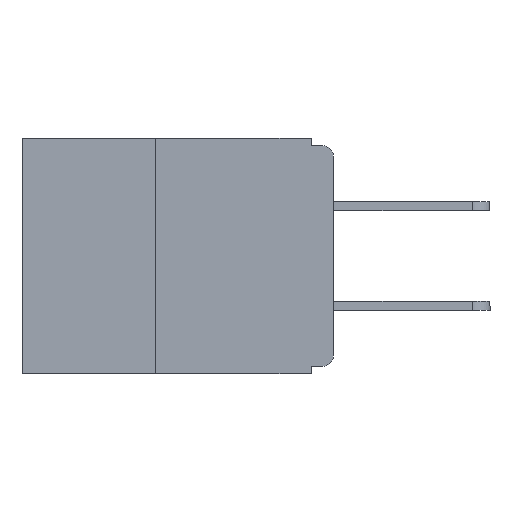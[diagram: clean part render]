
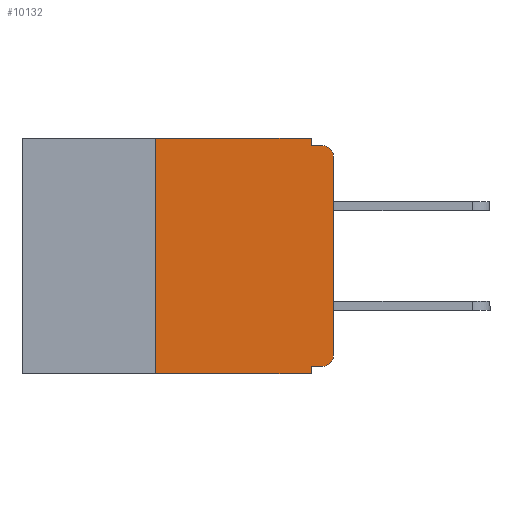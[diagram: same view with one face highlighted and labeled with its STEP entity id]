
A CAD part, left-side view. The second image highlights one B-rep face of the part: STEP entity #10132.
In plain terms, the highlighted planar face has unit normal (-1, 0, 0).
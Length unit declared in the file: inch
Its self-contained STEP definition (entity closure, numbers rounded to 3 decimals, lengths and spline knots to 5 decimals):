
#127 = LINE ( 'NONE', #15783, #6405 ) ;
#348 = VERTEX_POINT ( 'NONE', #14141 ) ;
#1384 = LINE ( 'NONE', #26669, #18188 ) ;
#2571 = CIRCLE ( 'NONE', #19677, 0.015 ) ;
#2648 = VERTEX_POINT ( 'NONE', #5834 ) ;
#2843 = DIRECTION ( 'NONE',  ( 1., 0., 0. ) ) ;
#3159 = EDGE_CURVE ( 'NONE', #17202, #8400, #13099, .T. ) ;
#3169 = AXIS2_PLACEMENT_3D ( 'NONE', #24977, #12440, #27015 ) ;
#4123 = DIRECTION ( 'NONE',  ( 0., 0., 1. ) ) ;
#4272 = LINE ( 'NONE', #15390, #20391 ) ;
#5052 = LINE ( 'NONE', #18734, #15496 ) ;
#5368 = DIRECTION ( 'NONE',  ( 0., -1., 0. ) ) ;
#5501 = CARTESIAN_POINT ( 'NONE',  ( 0., 0.031, -0.32 ) ) ;
#5834 = CARTESIAN_POINT ( 'NONE',  ( 0., 0.015, -0.32 ) ) ;
#6405 = VECTOR ( 'NONE', #5368, 39.37008 ) ;
#6448 = EDGE_CURVE ( 'NONE', #2648, #16755, #1384, .T. ) ;
#6973 = DIRECTION ( 'NONE',  ( 0., 0., -1. ) ) ;
#7498 = ORIENTED_EDGE ( 'NONE', *, *, #3159, .T. ) ;
#7514 = VERTEX_POINT ( 'NONE', #11996 ) ;
#7609 = ORIENTED_EDGE ( 'NONE', *, *, #23873, .T. ) ;
#7695 = CARTESIAN_POINT ( 'NONE',  ( 0., 0.031, 0. ) ) ;
#8369 = ORIENTED_EDGE ( 'NONE', *, *, #14883, .F. ) ;
#8400 = VERTEX_POINT ( 'NONE', #19944 ) ;
#8676 = DIRECTION ( 'NONE',  ( -1., 0., 0. ) ) ;
#9037 = CARTESIAN_POINT ( 'NONE',  ( 0., 0.437, 0. ) ) ;
#9240 = ORIENTED_EDGE ( 'NONE', *, *, #21764, .F. ) ;
#9447 = VECTOR ( 'NONE', #22319, 39.37008 ) ;
#9694 = ORIENTED_EDGE ( 'NONE', *, *, #19086, .F. ) ;
#10132 = ADVANCED_FACE ( 'NONE', ( #12997 ), #15371, .F. ) ;
#10397 = ORIENTED_EDGE ( 'NONE', *, *, #17545, .F. ) ;
#10726 = ORIENTED_EDGE ( 'NONE', *, *, #16083, .T. ) ;
#10773 = VERTEX_POINT ( 'NONE', #19555 ) ;
#11553 = CARTESIAN_POINT ( 'NONE',  ( 0., 0.437, 0. ) ) ;
#11996 = CARTESIAN_POINT ( 'NONE',  ( 0., 0.25, 0. ) ) ;
#12440 = DIRECTION ( 'NONE',  ( -1., 0., 0. ) ) ;
#12457 = ORIENTED_EDGE ( 'NONE', *, *, #14672, .F. ) ;
#12593 = ORIENTED_EDGE ( 'NONE', *, *, #6448, .F. ) ;
#12857 = ORIENTED_EDGE ( 'NONE', *, *, #21117, .T. ) ;
#12874 = CARTESIAN_POINT ( 'NONE',  ( 0., 0.031, 0. ) ) ;
#12969 = DIRECTION ( 'NONE',  ( 0., 0., -1. ) ) ;
#12997 = FACE_OUTER_BOUND ( 'NONE', #22557, .T. ) ;
#13099 = LINE ( 'NONE', #14351, #23636 ) ;
#13327 = VECTOR ( 'NONE', #12969, 39.37008 ) ;
#13436 = CARTESIAN_POINT ( 'NONE',  ( 0., 0., -0.305 ) ) ;
#14141 = CARTESIAN_POINT ( 'NONE',  ( 0., 0.031, -0.01 ) ) ;
#14351 = CARTESIAN_POINT ( 'NONE',  ( 0., 0., 0. ) ) ;
#14672 = EDGE_CURVE ( 'NONE', #16755, #25294, #4272, .T. ) ;
#14883 = EDGE_CURVE ( 'NONE', #348, #10773, #26150, .T. ) ;
#15371 = PLANE ( 'NONE',  #25863 ) ;
#15390 = CARTESIAN_POINT ( 'NONE',  ( 0., 0.031, -0.33 ) ) ;
#15496 = VECTOR ( 'NONE', #4123, 39.37008 ) ;
#15783 = CARTESIAN_POINT ( 'NONE',  ( 0., 0.437, -0.33 ) ) ;
#16023 = CARTESIAN_POINT ( 'NONE',  ( 0., 0., -0.01 ) ) ;
#16083 = EDGE_CURVE ( 'NONE', #18757, #25294, #127, .T. ) ;
#16755 = VERTEX_POINT ( 'NONE', #5501 ) ;
#17202 = VERTEX_POINT ( 'NONE', #13436 ) ;
#17540 = DIRECTION ( 'NONE',  ( 0., 0., -1. ) ) ;
#17545 = EDGE_CURVE ( 'NONE', #18757, #7514, #5052, .T. ) ;
#17796 = CIRCLE ( 'NONE', #3169, 0.015 ) ;
#17901 = DIRECTION ( 'NONE',  ( 0., -1., 0. ) ) ;
#18188 = VECTOR ( 'NONE', #26498, 39.37008 ) ;
#18734 = CARTESIAN_POINT ( 'NONE',  ( 0., 0.25, -0.33 ) ) ;
#18757 = VERTEX_POINT ( 'NONE', #21071 ) ;
#18991 = LINE ( 'NONE', #12874, #13327 ) ;
#19086 = EDGE_CURVE ( 'NONE', #7514, #20798, #22026, .T. ) ;
#19555 = CARTESIAN_POINT ( 'NONE',  ( 0., 0.015, -0.01 ) ) ;
#19677 = AXIS2_PLACEMENT_3D ( 'NONE', #21311, #8676, #23404 ) ;
#19944 = CARTESIAN_POINT ( 'NONE',  ( 0., 0., -0.025 ) ) ;
#20391 = VECTOR ( 'NONE', #6973, 39.37008 ) ;
#20798 = VERTEX_POINT ( 'NONE', #7695 ) ;
#21071 = CARTESIAN_POINT ( 'NONE',  ( 0., 0.25, -0.33 ) ) ;
#21117 = EDGE_CURVE ( 'NONE', #2648, #17202, #2571, .T. ) ;
#21311 = CARTESIAN_POINT ( 'NONE',  ( 0., 0.015, -0.305 ) ) ;
#21400 = VECTOR ( 'NONE', #17901, 39.37008 ) ;
#21499 = CARTESIAN_POINT ( 'NONE',  ( 0., 0.031, -0.33 ) ) ;
#21764 = EDGE_CURVE ( 'NONE', #20798, #348, #18991, .T. ) ;
#22026 = LINE ( 'NONE', #11553, #21400 ) ;
#22319 = DIRECTION ( 'NONE',  ( 0., -1., 0. ) ) ;
#22557 = EDGE_LOOP ( 'NONE', ( #7498, #7609, #8369, #9240, #9694, #10397, #10726, #12457, #12593, #12857 ) ) ;
#23404 = DIRECTION ( 'NONE',  ( 0., 0., -1. ) ) ;
#23636 = VECTOR ( 'NONE', #26063, 39.37008 ) ;
#23873 = EDGE_CURVE ( 'NONE', #8400, #10773, #17796, .T. ) ;
#24977 = CARTESIAN_POINT ( 'NONE',  ( 0., 0.015, -0.025 ) ) ;
#25294 = VERTEX_POINT ( 'NONE', #21499 ) ;
#25863 = AXIS2_PLACEMENT_3D ( 'NONE', #9037, #2843, #17540 ) ;
#26063 = DIRECTION ( 'NONE',  ( 0., 0., 1. ) ) ;
#26150 = LINE ( 'NONE', #16023, #9447 ) ;
#26498 = DIRECTION ( 'NONE',  ( 0., 1., 0. ) ) ;
#26669 = CARTESIAN_POINT ( 'NONE',  ( 0., 0., -0.32 ) ) ;
#27015 = DIRECTION ( 'NONE',  ( 0., 0., -1. ) ) ;
